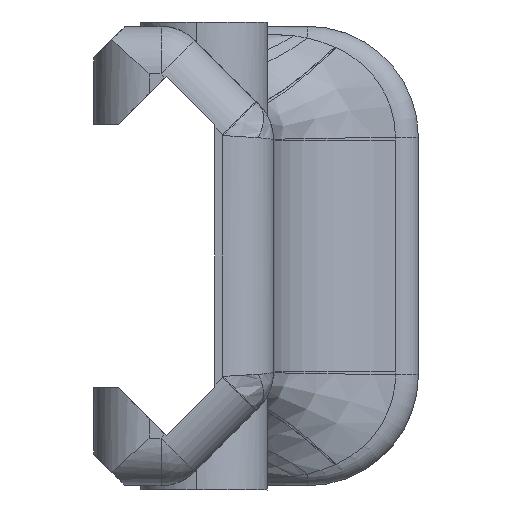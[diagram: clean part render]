
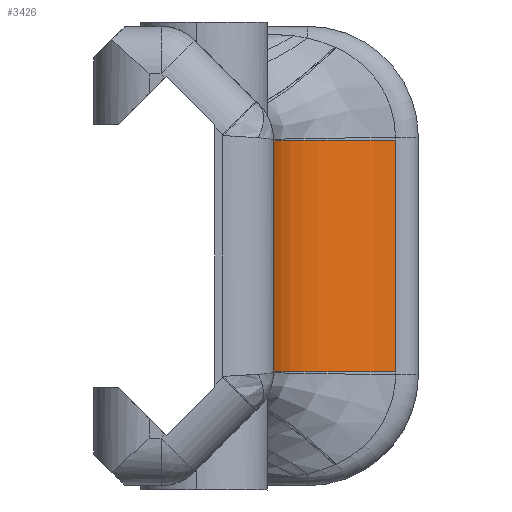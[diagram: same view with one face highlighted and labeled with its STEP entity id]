
A CAD part, left-side view. The second image highlights one B-rep face of the part: STEP entity #3426.
In plain terms, the highlighted cylindrical face has radius 8 mm (diameter 16 mm), a partial arc.
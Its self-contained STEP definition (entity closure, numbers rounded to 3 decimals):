
#129=LINE('',#5012,#325);
#306=LINE('',#7554,#502);
#325=VECTOR('',#3835,10.);
#502=VECTOR('',#4534,10.);
#559=CYLINDRICAL_SURFACE('',#3747,8.);
#831=FACE_OUTER_BOUND('',#1041,.T.);
#1041=EDGE_LOOP('',(#3138,#3139,#3140,#3141));
#1161=CIRCLE('',#3723,8.);
#1173=CIRCLE('',#3748,8.);
#1389=VERTEX_POINT('',#4983);
#1392=VERTEX_POINT('',#5007);
#1639=VERTEX_POINT('',#7296);
#1654=VERTEX_POINT('',#7548);
#1725=EDGE_CURVE('',#1389,#1392,#129,.T.);
#2128=EDGE_CURVE('',#1639,#1389,#1161,.T.);
#2159=EDGE_CURVE('',#1654,#1639,#306,.T.);
#2160=EDGE_CURVE('',#1654,#1392,#1173,.T.);
#3138=ORIENTED_EDGE('',*,*,#2128,.T.);
#3139=ORIENTED_EDGE('',*,*,#1725,.T.);
#3140=ORIENTED_EDGE('',*,*,#2160,.F.);
#3141=ORIENTED_EDGE('',*,*,#2159,.T.);
#3426=ADVANCED_FACE('',(#831),#559,.F.);
#3723=AXIS2_PLACEMENT_3D('',#7297,#4482,#4483);
#3747=AXIS2_PLACEMENT_3D('',#7555,#4535,#4536);
#3748=AXIS2_PLACEMENT_3D('',#7556,#4537,#4538);
#3835=DIRECTION('',(0.,0.,-1.));
#4482=DIRECTION('center_axis',(0.,0.,
1.));
#4483=DIRECTION('ref_axis',(0.999,0.037,0.));
#4534=DIRECTION('',(0.,0.,1.));
#4535=DIRECTION('center_axis',(0.,0.,
1.));
#4536=DIRECTION('ref_axis',(0.694,0.72,0.));
#4537=DIRECTION('center_axis',(0.,0.,
1.));
#4538=DIRECTION('ref_axis',(0.999,0.037,0.));
#4983=CARTESIAN_POINT('',(-7.613,-43.078,11.112));
#5007=CARTESIAN_POINT('',(-7.613,-43.077,-3.529));
#5012=CARTESIAN_POINT('',(-7.613,-43.077,-3.458));
#7296=CARTESIAN_POINT('',(0.381,-50.779,11.112));
#7297=CARTESIAN_POINT('Origin',(-7.613,-51.078,11.112));
#7548=CARTESIAN_POINT('',(0.381,-50.779,-3.529));
#7554=CARTESIAN_POINT('',(0.381,-50.779,-3.458));
#7555=CARTESIAN_POINT('Origin',(-7.613,-51.077,-3.459));
#7556=CARTESIAN_POINT('Origin',(-7.613,-51.077,-3.529));
